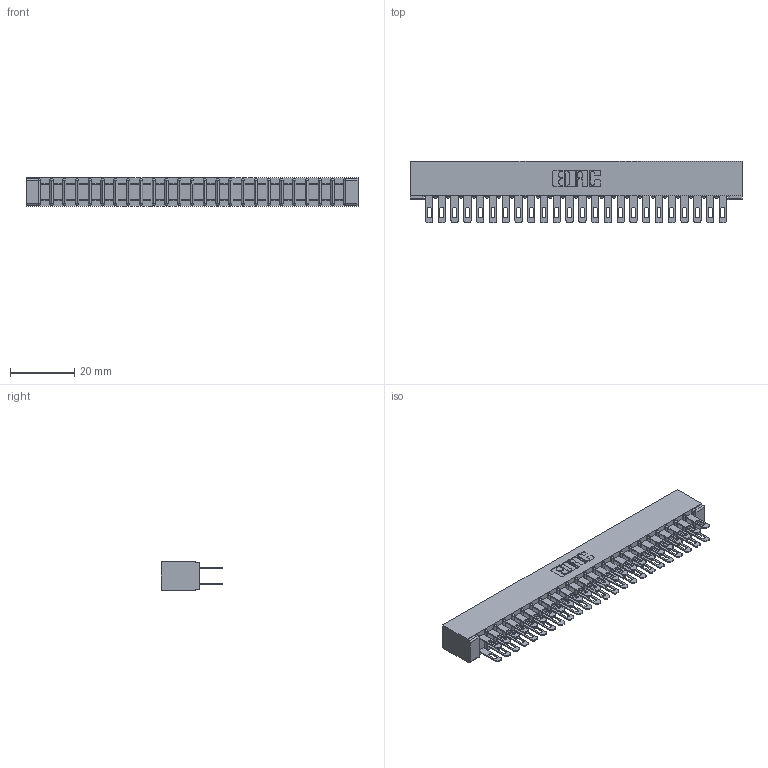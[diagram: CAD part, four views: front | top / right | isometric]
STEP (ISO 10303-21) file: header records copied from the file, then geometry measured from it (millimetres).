
FILE_DESCRIPTION (( 'STEP AP203' ), '1' );
FILE_NAME ('357-048-500-201.STEP', '2018-08-11T13:38:09', ( '' ), ( '' ), 'SwSTEP 2.0', 'SolidWorks 2016', '' );
FILE_SCHEMA (( 'CONFIG_CONTROL_DESIGN' ));
Length unit declared in the file: inch
Products named in the file (3): 307 Part_No Mounting Lugs; 307-290-001_500; 357-048-500-201
Assembly tree (49 placements, depth 2):
  357-048-500-201
    307 Part_No Mounting Lugs
    307-290-001_500  x48
Bounding box: 102.97 x 19.18 x 8.71 mm (x, y, z)
Volume: 7105.9 mm3; surface area: 13888.6 mm2
Topology: 49 solids, 49 shells, 2343 faces, 6539 edges, 4226 vertices
Faces by surface type: plane 1506, cylinder 787, sphere 50
Entity records: 23258 total; most frequent: CARTESIAN_POINT 3804, ORIENTED_EDGE 3766, DIRECTION 3735, EDGE_CURVE 1883, VECTOR 1437, LINE 1437, VERTEX_POINT 1218, AXIS2_PLACEMENT_3D 1149
